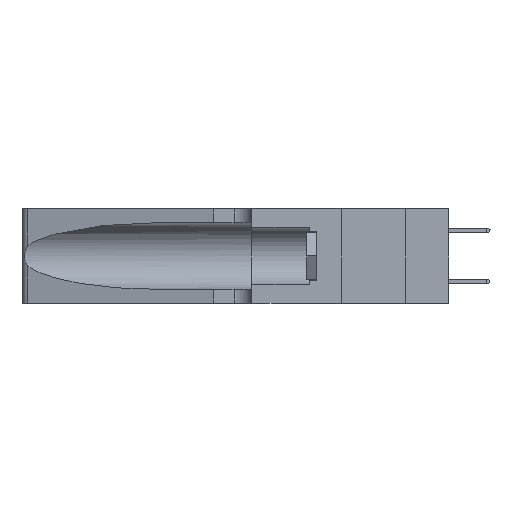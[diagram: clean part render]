
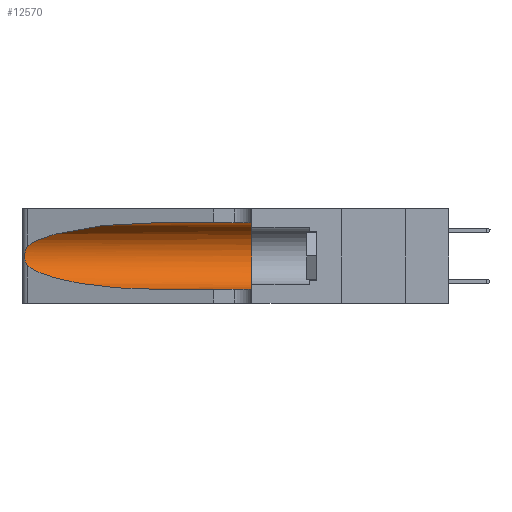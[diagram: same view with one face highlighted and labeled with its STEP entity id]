
A CAD part, left-side view. The second image highlights one B-rep face of the part: STEP entity #12570.
In plain terms, the highlighted cylindrical face has radius 3.308 mm (diameter 6.617 mm), a partial arc.
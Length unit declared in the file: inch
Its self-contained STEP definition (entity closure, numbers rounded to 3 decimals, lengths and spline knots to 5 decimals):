
#180 = ORIENTED_EDGE ( 'NONE', *, *, #33777, .T. ) ;
#184 = AXIS2_PLACEMENT_3D ( 'NONE', #31273, #2724, #5476 ) ;
#191 = CARTESIAN_POINT ( 'NONE',  ( 0.26017, 1.23833, 0.17102 ) ) ;
#2724 = DIRECTION ( 'NONE',  ( 0., 1., 0. ) ) ;
#2893 = ORIENTED_EDGE ( 'NONE', *, *, #40386, .F. ) ;
#2980 = CARTESIAN_POINT ( 'NONE',  ( 0.25787, 1.23484, 0.2124 ) ) ;
#3111 = CYLINDRICAL_SURFACE ( 'NONE', #11607, 0.13025 ) ;
#4194 = VECTOR ( 'NONE', #9198, 39.37008 ) ;
#5450 = CIRCLE ( 'NONE', #184, 0.13025 ) ;
#5476 = DIRECTION ( 'NONE',  ( 0., 0., 1. ) ) ;
#5592 = CARTESIAN_POINT ( 'NONE',  ( 0.1305, 0.72297, 0.05475 ) ) ;
#5620 = CARTESIAN_POINT ( 'NONE',  ( 0.25555, 1.22994, 0.2215 ) ) ;
#7498 = ORIENTED_EDGE ( 'NONE', *, *, #22630, .F. ) ;
#9078 = FACE_OUTER_BOUND ( 'NONE', #24880, .T. ) ;
#9198 = DIRECTION ( 'NONE',  ( 0., -1., 0. ) ) ;
#9359 = CARTESIAN_POINT ( 'NONE',  ( 0.26075, 1.23896, 0.19203 ) ) ;
#10629 = CARTESIAN_POINT ( 'NONE',  ( 0.2373, 1.15595, 0.28018 ) ) ;
#10764 = CARTESIAN_POINT ( 'NONE',  ( 0.25487, 1.22718, 0.22369 ) ) ;
#11295 = VECTOR ( 'NONE', #22813, 39.37008 ) ;
#11607 = AXIS2_PLACEMENT_3D ( 'NONE', #29329, #29051, #22804 ) ;
#11852 = CARTESIAN_POINT ( 'NONE',  ( 0.1305, 1.61858, 0.05475 ) ) ;
#12375 = VERTEX_POINT ( 'NONE', #25471 ) ;
#12570 = ADVANCED_FACE ( 'NONE', ( #9078 ), #3111, .F. ) ;
#13470 = EDGE_CURVE ( 'NONE', #12375, #24472, #38250, .T. ) ;
#13523 = CARTESIAN_POINT ( 'NONE',  ( 0.25487, 1.22718, 0.14631 ) ) ;
#14255 = CARTESIAN_POINT ( 'NONE',  ( 0.1305, 0.72297, 0.31525 ) ) ;
#14710 = CARTESIAN_POINT ( 'NONE',  ( 0.25487, 1.22718, 0.14631 ) ) ;
#16101 = CARTESIAN_POINT ( 'NONE',  ( 0.1305, 0.72297, 0.31525 ) ) ;
#16875 = ORIENTED_EDGE ( 'NONE', *, *, #13470, .T. ) ;
#19062 = CARTESIAN_POINT ( 'NONE',  ( 0.1305, 1.61858, 0.31525 ) ) ;
#19782 = CARTESIAN_POINT ( 'NONE',  ( 0.25639, 1.23186, 0.15144 ) ) ;
#19921 = CARTESIAN_POINT ( 'NONE',  ( 0.25555, 1.22993, 0.14849 ) ) ;
#21002 = EDGE_CURVE ( 'NONE', #24472, #27409, #28342, .T. ) ;
#22443 =( BOUNDED_CURVE ( )  B_SPLINE_CURVE ( 3, ( #14255, #39004, #10629, #10764 ),
 .UNSPECIFIED., .F., .T. ) 
 B_SPLINE_CURVE_WITH_KNOTS ( ( 4, 4 ),
 ( 1.5708, 2.84003 ),
 .UNSPECIFIED. ) 
 CURVE ( )  GEOMETRIC_REPRESENTATION_ITEM ( )  RATIONAL_B_SPLINE_CURVE ( ( 1., 0.87, 0.87, 1. ) ) 
 REPRESENTATION_ITEM ( '' )  );
#22630 = EDGE_CURVE ( 'NONE', #30414, #29379, #26743, .T. ) ;
#22731 = CARTESIAN_POINT ( 'NONE',  ( 0.25789, 1.23486, 0.15765 ) ) ;
#22804 = DIRECTION ( 'NONE',  ( 0., 0., -1. ) ) ;
#22813 = DIRECTION ( 'NONE',  ( 0., -1., 0. ) ) ;
#24472 = VERTEX_POINT ( 'NONE', #14710 ) ;
#24880 = EDGE_LOOP ( 'NONE', ( #30497, #16875, #26248, #180, #2893, #7498 ) ) ;
#25471 = CARTESIAN_POINT ( 'NONE',  ( 0.25487, 1.22718, 0.22369 ) ) ;
#26160 = VERTEX_POINT ( 'NONE', #32211 ) ;
#26248 = ORIENTED_EDGE ( 'NONE', *, *, #21002, .T. ) ;
#26743 = LINE ( 'NONE', #19062, #11295 ) ;
#26874 = CARTESIAN_POINT ( 'NONE',  ( 0.2373, 1.15595, 0.08982 ) ) ;
#27409 = VERTEX_POINT ( 'NONE', #28601 ) ;
#27543 = CARTESIAN_POINT ( 'NONE',  ( 0.1305, 0.35, 0.31525 ) ) ;
#28119 = LINE ( 'NONE', #11852, #4194 ) ;
#28342 =( BOUNDED_CURVE ( )  B_SPLINE_CURVE ( 3, ( #30272, #26874, #33887, #5592 ),
 .UNSPECIFIED., .F., .F. ) 
 B_SPLINE_CURVE_WITH_KNOTS ( ( 4, 4 ),
 ( 3.44316, 4.71239 ),
 .UNSPECIFIED. ) 
 CURVE ( )  GEOMETRIC_REPRESENTATION_ITEM ( )  RATIONAL_B_SPLINE_CURVE ( ( 1., 0.87, 0.87, 1. ) ) 
 REPRESENTATION_ITEM ( '' )  );
#28601 = CARTESIAN_POINT ( 'NONE',  ( 0.1305, 0.72297, 0.05475 ) ) ;
#29051 = DIRECTION ( 'NONE',  ( 0., -1., 0. ) ) ;
#29329 = CARTESIAN_POINT ( 'NONE',  ( 0.1305, 1.61858, 0.185 ) ) ;
#29379 = VERTEX_POINT ( 'NONE', #27543 ) ;
#29538 = CARTESIAN_POINT ( 'NONE',  ( 0.25856, 1.23593, 0.16098 ) ) ;
#30272 = CARTESIAN_POINT ( 'NONE',  ( 0.25487, 1.22718, 0.14631 ) ) ;
#30414 = VERTEX_POINT ( 'NONE', #16101 ) ;
#30497 = ORIENTED_EDGE ( 'NONE', *, *, #32607, .T. ) ;
#31273 = CARTESIAN_POINT ( 'NONE',  ( 0.1305, 0.35, 0.185 ) ) ;
#31933 = CARTESIAN_POINT ( 'NONE',  ( 0.26018, 1.23835, 0.19895 ) ) ;
#32211 = CARTESIAN_POINT ( 'NONE',  ( 0.1305, 0.35, 0.05475 ) ) ;
#32607 = EDGE_CURVE ( 'NONE', #30414, #12375, #22443, .T. ) ;
#33777 = EDGE_CURVE ( 'NONE', #27409, #26160, #28119, .T. ) ;
#33887 = CARTESIAN_POINT ( 'NONE',  ( 0.18966, 0.96281, 0.05475 ) ) ;
#37756 = CARTESIAN_POINT ( 'NONE',  ( 0.25487, 1.22718, 0.22369 ) ) ;
#38021 = CARTESIAN_POINT ( 'NONE',  ( 0.26075, 1.23896, 0.178 ) ) ;
#38250 = B_SPLINE_CURVE_WITH_KNOTS ( 'NONE', 3,
 ( #37756, #5620, #41090, #2980, #38280, #31933, #9359, #38021, #191, #29538, #22731, #19782, #19921, #13523 ),
 .UNSPECIFIED., .F., .F.,
 ( 4, 2, 2, 2, 2, 2, 4 ),
 ( 0., 0.00027, 0.00053, 0.00107, 0.0016, 0.00187, 0.00214 ),
 .UNSPECIFIED. ) ;
#38280 = CARTESIAN_POINT ( 'NONE',  ( 0.25854, 1.2359, 0.20912 ) ) ;
#39004 = CARTESIAN_POINT ( 'NONE',  ( 0.18966, 0.96281, 0.31525 ) ) ;
#40386 = EDGE_CURVE ( 'NONE', #29379, #26160, #5450, .T. ) ;
#41090 = CARTESIAN_POINT ( 'NONE',  ( 0.25639, 1.23184, 0.21858 ) ) ;
